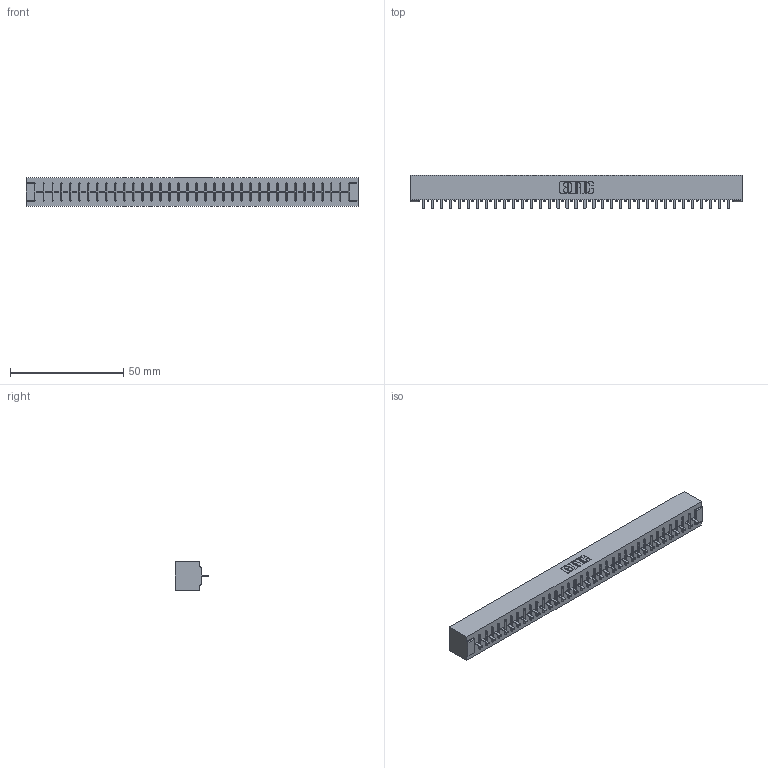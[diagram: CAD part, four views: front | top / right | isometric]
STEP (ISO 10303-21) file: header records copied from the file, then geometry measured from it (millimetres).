
FILE_DESCRIPTION (( 'STEP AP203' ), '1' );
FILE_NAME ('316-035-421-101.STEP', '2020-09-23T04:44:15', ( '' ), ( '' ), 'SwSTEP 2.0', 'SolidWorks 2020', '' );
FILE_SCHEMA (( 'CONFIG_CONTROL_DESIGN' ));
Length unit declared in the file: inch
Products named in the file (3): 306 Part_No Mounting; 306-290-001_121; 316-035-421-101
Assembly tree (36 placements, depth 2):
  316-035-421-101
    306 Part_No Mounting
    306-290-001_121  x35
Bounding box: 146.56 x 14.88 x 12.7 mm (x, y, z)
Volume: 16684.8 mm3; surface area: 16924.2 mm2
Topology: 36 solids, 36 shells, 2558 faces, 7187 edges, 4602 vertices
Faces by surface type: plane 1709, cylinder 709, sphere 140
Entity records: 33224 total; most frequent: CARTESIAN_POINT 5576, ORIENTED_EDGE 5526, DIRECTION 5499, EDGE_CURVE 2763, VECTOR 2161, LINE 2161, VERTEX_POINT 1746, AXIS2_PLACEMENT_3D 1669
